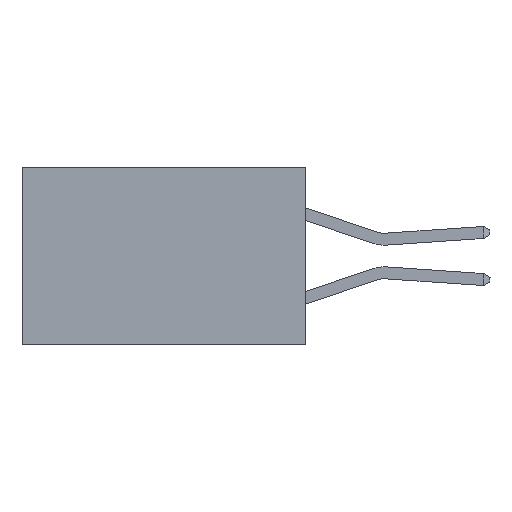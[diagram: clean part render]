
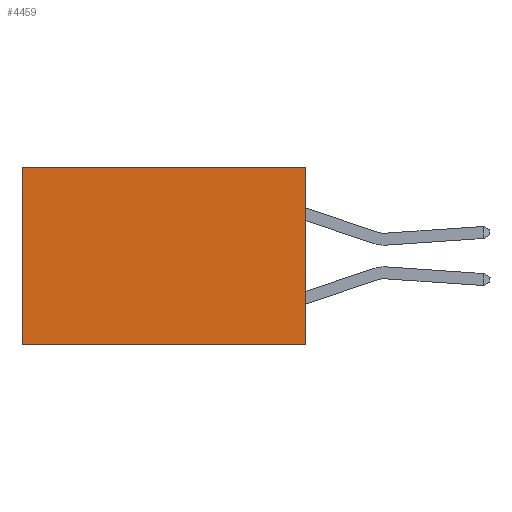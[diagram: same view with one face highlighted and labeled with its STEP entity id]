
A CAD part, left-side view. The second image highlights one B-rep face of the part: STEP entity #4459.
In plain terms, the highlighted planar face has unit normal (-1, 0, 0).
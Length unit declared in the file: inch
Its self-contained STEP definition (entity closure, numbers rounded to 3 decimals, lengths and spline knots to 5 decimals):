
#370 = EDGE_CURVE ( 'NONE', #1686, #10303, #8924, .T. ) ;
#639 = DIRECTION ( 'NONE',  ( 0., 1., 0. ) ) ;
#1322 = CARTESIAN_POINT ( 'NONE',  ( 0.277, 0., -0.37 ) ) ;
#1378 = CARTESIAN_POINT ( 'NONE',  ( 0.277, 0.59, 0. ) ) ;
#1678 = CARTESIAN_POINT ( 'NONE',  ( 0.277, 0., 0. ) ) ;
#1686 = VERTEX_POINT ( 'NONE', #1378 ) ;
#1838 = CARTESIAN_POINT ( 'NONE',  ( 0.277, 0., -0.37 ) ) ;
#2142 = VECTOR ( 'NONE', #10704, 39.37008 ) ;
#2533 = EDGE_CURVE ( 'NONE', #8375, #9257, #9773, .T. ) ;
#3457 = LINE ( 'NONE', #5243, #7902 ) ;
#3507 = PLANE ( 'NONE',  #9386 ) ;
#4081 = ORIENTED_EDGE ( 'NONE', *, *, #370, .T. ) ;
#4139 = ORIENTED_EDGE ( 'NONE', *, *, #4415, .F. ) ;
#4245 = ORIENTED_EDGE ( 'NONE', *, *, #2533, .F. ) ;
#4415 = EDGE_CURVE ( 'NONE', #9257, #10303, #7294, .T. ) ;
#4459 = ADVANCED_FACE ( 'NONE', ( #8971 ), #3507, .F. ) ;
#4588 = ORIENTED_EDGE ( 'NONE', *, *, #10267, .T. ) ;
#4910 = EDGE_LOOP ( 'NONE', ( #4081, #4139, #4245, #4588 ) ) ;
#4971 = VECTOR ( 'NONE', #6090, 39.37008 ) ;
#4990 = CARTESIAN_POINT ( 'NONE',  ( 0.277, 0., -0.37 ) ) ;
#5243 = CARTESIAN_POINT ( 'NONE',  ( 0.277, 0., 0. ) ) ;
#6090 = DIRECTION ( 'NONE',  ( 0., 1., 0. ) ) ;
#6186 = CARTESIAN_POINT ( 'NONE',  ( 0.277, 0.59, -0.37 ) ) ;
#6994 = CARTESIAN_POINT ( 'NONE',  ( 0.277, 0.59, -0.37 ) ) ;
#7294 = LINE ( 'NONE', #4990, #4971 ) ;
#7592 = VECTOR ( 'NONE', #9586, 39.37008 ) ;
#7902 = VECTOR ( 'NONE', #639, 39.37008 ) ;
#8375 = VERTEX_POINT ( 'NONE', #1678 ) ;
#8924 = LINE ( 'NONE', #6994, #2142 ) ;
#8971 = FACE_OUTER_BOUND ( 'NONE', #4910, .T. ) ;
#9167 = CARTESIAN_POINT ( 'NONE',  ( 0.277, 0., -0.37 ) ) ;
#9257 = VERTEX_POINT ( 'NONE', #1322 ) ;
#9386 = AXIS2_PLACEMENT_3D ( 'NONE', #9167, #10385, #9605 ) ;
#9586 = DIRECTION ( 'NONE',  ( 0., 0., -1. ) ) ;
#9605 = DIRECTION ( 'NONE',  ( 0., 0., -1. ) ) ;
#9773 = LINE ( 'NONE', #1838, #7592 ) ;
#10267 = EDGE_CURVE ( 'NONE', #8375, #1686, #3457, .T. ) ;
#10303 = VERTEX_POINT ( 'NONE', #6186 ) ;
#10385 = DIRECTION ( 'NONE',  ( 1., 0., 0. ) ) ;
#10704 = DIRECTION ( 'NONE',  ( 0., 0., -1. ) ) ;
